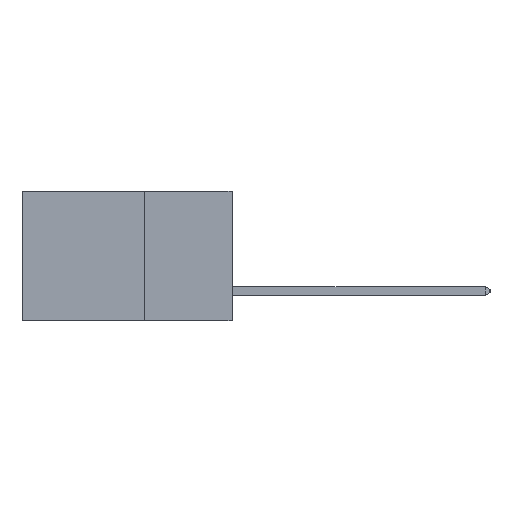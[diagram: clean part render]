
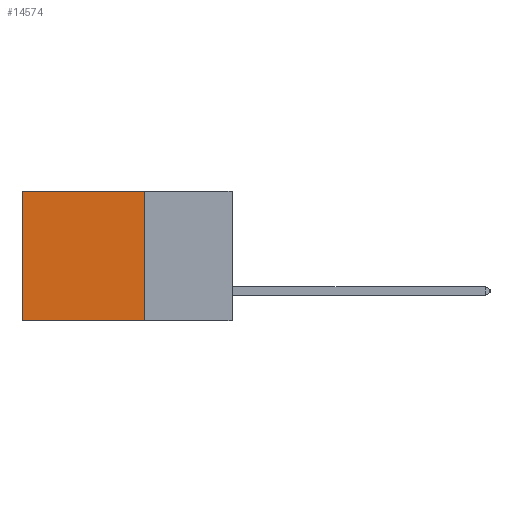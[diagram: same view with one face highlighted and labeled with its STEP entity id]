
A CAD part, left-side view. The second image highlights one B-rep face of the part: STEP entity #14574.
In plain terms, the highlighted planar face has unit normal (-1, 0, 0).
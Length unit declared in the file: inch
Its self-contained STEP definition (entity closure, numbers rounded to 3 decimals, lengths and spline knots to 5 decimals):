
#43 = CARTESIAN_POINT ( 'NONE',  ( 0.2875, 0.25, 0. ) ) ;
#638 = CARTESIAN_POINT ( 'NONE',  ( 0.2875, 0.6, -0.37 ) ) ;
#1549 = CARTESIAN_POINT ( 'NONE',  ( 0.2875, 0.25, 0. ) ) ;
#1565 = CARTESIAN_POINT ( 'NONE',  ( 0.2875, 0.25, 0. ) ) ;
#2279 = EDGE_CURVE ( 'NONE', #4615, #5243, #14405, .T. ) ;
#2900 = EDGE_CURVE ( 'NONE', #4615, #20267, #19401, .T. ) ;
#3956 = DIRECTION ( 'NONE',  ( 0., 1., 0. ) ) ;
#4327 = CARTESIAN_POINT ( 'NONE',  ( 0.2875, 0.25, 0. ) ) ;
#4615 = VERTEX_POINT ( 'NONE', #1549 ) ;
#5243 = VERTEX_POINT ( 'NONE', #14402 ) ;
#5402 = VECTOR ( 'NONE', #11503, 39.37008 ) ;
#5488 = AXIS2_PLACEMENT_3D ( 'NONE', #4327, #15567, #6012 ) ;
#5718 = CARTESIAN_POINT ( 'NONE',  ( 0.2875, 0.6, 0. ) ) ;
#6012 = DIRECTION ( 'NONE',  ( 0., 0., -1. ) ) ;
#6149 = VECTOR ( 'NONE', #17713, 39.37008 ) ;
#6252 = VERTEX_POINT ( 'NONE', #638 ) ;
#8013 = EDGE_LOOP ( 'NONE', ( #19604, #18955, #17319, #14063 ) ) ;
#10283 = FACE_OUTER_BOUND ( 'NONE', #8013, .T. ) ;
#10332 = CARTESIAN_POINT ( 'NONE',  ( 0.2875, 0.6, 0. ) ) ;
#11503 = DIRECTION ( 'NONE',  ( 0., 0., -1. ) ) ;
#12022 = CARTESIAN_POINT ( 'NONE',  ( 0.2875, 0.25, -0.37 ) ) ;
#12281 = VECTOR ( 'NONE', #3956, 39.37008 ) ;
#12373 = PLANE ( 'NONE',  #5488 ) ;
#13267 = LINE ( 'NONE', #12022, #12281 ) ;
#14063 = ORIENTED_EDGE ( 'NONE', *, *, #2900, .T. ) ;
#14402 = CARTESIAN_POINT ( 'NONE',  ( 0.2875, 0.25, -0.37 ) ) ;
#14405 = LINE ( 'NONE', #43, #5402 ) ;
#14574 = ADVANCED_FACE ( 'NONE', ( #10283 ), #12373, .F. ) ;
#15567 = DIRECTION ( 'NONE',  ( 1., 0., 0. ) ) ;
#16165 = EDGE_CURVE ( 'NONE', #20267, #6252, #18290, .T. ) ;
#16683 = DIRECTION ( 'NONE',  ( 0., 0., -1. ) ) ;
#16837 = EDGE_CURVE ( 'NONE', #5243, #6252, #13267, .T. ) ;
#17319 = ORIENTED_EDGE ( 'NONE', *, *, #2279, .F. ) ;
#17713 = DIRECTION ( 'NONE',  ( 0., 1., 0. ) ) ;
#17789 = VECTOR ( 'NONE', #16683, 39.37008 ) ;
#18290 = LINE ( 'NONE', #10332, #17789 ) ;
#18955 = ORIENTED_EDGE ( 'NONE', *, *, #16837, .F. ) ;
#19401 = LINE ( 'NONE', #1565, #6149 ) ;
#19604 = ORIENTED_EDGE ( 'NONE', *, *, #16165, .T. ) ;
#20267 = VERTEX_POINT ( 'NONE', #5718 ) ;
